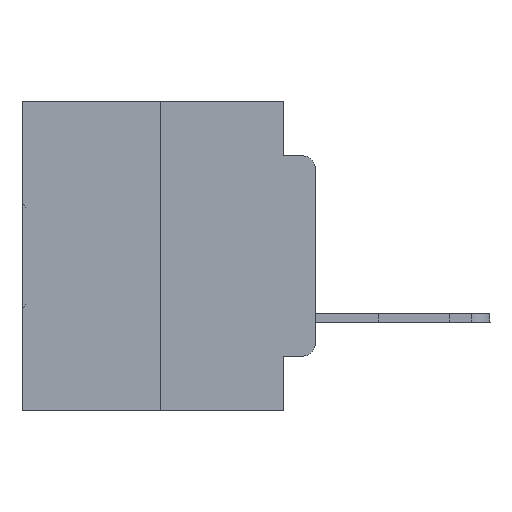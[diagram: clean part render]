
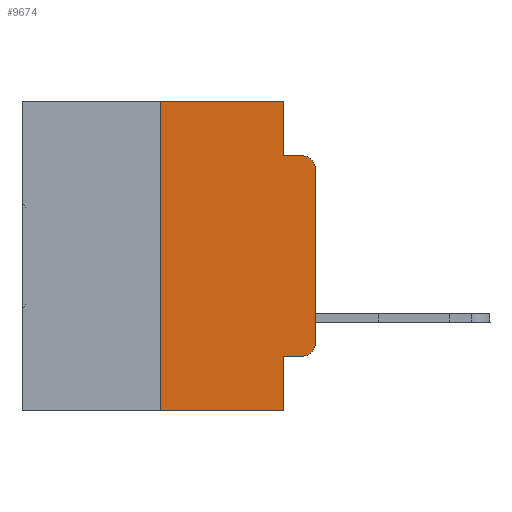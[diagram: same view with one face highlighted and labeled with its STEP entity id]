
A CAD part, left-side view. The second image highlights one B-rep face of the part: STEP entity #9674.
In plain terms, the highlighted planar face has unit normal (-1, 0, 0).
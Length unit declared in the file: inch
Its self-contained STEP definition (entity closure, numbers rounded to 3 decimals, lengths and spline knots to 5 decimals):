
#118 = ORIENTED_EDGE ( 'NONE', *, *, #8138, .T. ) ;
#133 = LINE ( 'NONE', #28961, #28469 ) ;
#849 = DIRECTION ( 'NONE',  ( -1., 0., 0. ) ) ;
#954 = DIRECTION ( 'NONE',  ( 0., 0., -1. ) ) ;
#1619 = CARTESIAN_POINT ( 'NONE',  ( 0., 0.473, 0. ) ) ;
#2212 = FACE_OUTER_BOUND ( 'NONE', #28470, .T. ) ;
#2397 = ORIENTED_EDGE ( 'NONE', *, *, #27612, .T. ) ;
#2568 = CIRCLE ( 'NONE', #22757, 0.02 ) ;
#2990 = VECTOR ( 'NONE', #17232, 39.37008 ) ;
#3203 = EDGE_CURVE ( 'NONE', #25493, #4615, #4268, .T. ) ;
#4016 = CARTESIAN_POINT ( 'NONE',  ( 0., 0.02, -0.4115 ) ) ;
#4268 = LINE ( 'NONE', #20964, #20093 ) ;
#4605 = VERTEX_POINT ( 'NONE', #16360 ) ;
#4615 = VERTEX_POINT ( 'NONE', #11891 ) ;
#5071 = VECTOR ( 'NONE', #20044, 39.37008 ) ;
#5284 = CARTESIAN_POINT ( 'NONE',  ( 0., 0.051, 0. ) ) ;
#5314 = EDGE_CURVE ( 'NONE', #11670, #20157, #16582, .T. ) ;
#5320 = ORIENTED_EDGE ( 'NONE', *, *, #5314, .T. ) ;
#6007 = CARTESIAN_POINT ( 'NONE',  ( 0., 0., -0.1085 ) ) ;
#6512 = DIRECTION ( 'NONE',  ( 0., 0., 1. ) ) ;
#6536 = VERTEX_POINT ( 'NONE', #9984 ) ;
#6671 = VERTEX_POINT ( 'NONE', #12027 ) ;
#7410 = CIRCLE ( 'NONE', #23079, 0.02 ) ;
#7825 = CARTESIAN_POINT ( 'NONE',  ( 0., 0.02, -0.1085 ) ) ;
#7965 = DIRECTION ( 'NONE',  ( 0., 0., -1. ) ) ;
#8040 = DIRECTION ( 'NONE',  ( 0., -1., 0. ) ) ;
#8138 = EDGE_CURVE ( 'NONE', #6536, #22049, #23464, .T. ) ;
#8354 = EDGE_CURVE ( 'NONE', #6671, #29490, #18527, .T. ) ;
#8698 = CARTESIAN_POINT ( 'NONE',  ( 0., 0.051, -0.5 ) ) ;
#8813 = DIRECTION ( 'NONE',  ( 0., -1., 0. ) ) ;
#9592 = EDGE_CURVE ( 'NONE', #20157, #6536, #2568, .T. ) ;
#9674 = ADVANCED_FACE ( 'NONE', ( #2212 ), #11490, .F. ) ;
#9708 = CARTESIAN_POINT ( 'NONE',  ( 0., 0., 0. ) ) ;
#9984 = CARTESIAN_POINT ( 'NONE',  ( 0., 0., -0.3915 ) ) ;
#10073 = DIRECTION ( 'NONE',  ( 0., -1., 0. ) ) ;
#10475 = VECTOR ( 'NONE', #8040, 39.37008 ) ;
#10512 = CARTESIAN_POINT ( 'NONE',  ( 0., 0.02, -0.3915 ) ) ;
#10734 = VERTEX_POINT ( 'NONE', #8698 ) ;
#10777 = CARTESIAN_POINT ( 'NONE',  ( 0., 0.051, -0.0885 ) ) ;
#10799 = DIRECTION ( 'NONE',  ( 1., 0., 0. ) ) ;
#10843 = AXIS2_PLACEMENT_3D ( 'NONE', #21805, #10799, #23010 ) ;
#11021 = ORIENTED_EDGE ( 'NONE', *, *, #9592, .T. ) ;
#11490 = PLANE ( 'NONE',  #10843 ) ;
#11670 = VERTEX_POINT ( 'NONE', #25630 ) ;
#11891 = CARTESIAN_POINT ( 'NONE',  ( 0., 0.25, 0. ) ) ;
#12027 = CARTESIAN_POINT ( 'NONE',  ( 0., 0.051, 0. ) ) ;
#13637 = LINE ( 'NONE', #15046, #2990 ) ;
#13674 = ORIENTED_EDGE ( 'NONE', *, *, #25780, .F. ) ;
#14343 = CARTESIAN_POINT ( 'NONE',  ( 0., 0.25, -0.5 ) ) ;
#14591 = ORIENTED_EDGE ( 'NONE', *, *, #18285, .F. ) ;
#15046 = CARTESIAN_POINT ( 'NONE',  ( 0., 0.473, -0.5 ) ) ;
#15161 = CARTESIAN_POINT ( 'NONE',  ( 0., 0.051, -0.4115 ) ) ;
#15295 = DIRECTION ( 'NONE',  ( -1., 0., 0. ) ) ;
#16360 = CARTESIAN_POINT ( 'NONE',  ( 0., 0.02, -0.0885 ) ) ;
#16582 = LINE ( 'NONE', #15161, #10475 ) ;
#16876 = VECTOR ( 'NONE', #8813, 39.37008 ) ;
#17232 = DIRECTION ( 'NONE',  ( 0., -1., 0. ) ) ;
#17324 = EDGE_CURVE ( 'NONE', #22049, #4605, #7410, .T. ) ;
#17903 = LINE ( 'NONE', #5284, #5071 ) ;
#18148 = VECTOR ( 'NONE', #7965, 39.37008 ) ;
#18285 = EDGE_CURVE ( 'NONE', #11670, #10734, #17903, .T. ) ;
#18527 = LINE ( 'NONE', #20007, #18148 ) ;
#19208 = DIRECTION ( 'NONE',  ( 0., 0., 1. ) ) ;
#20007 = CARTESIAN_POINT ( 'NONE',  ( 0., 0.051, 0. ) ) ;
#20044 = DIRECTION ( 'NONE',  ( 0., 0., -1. ) ) ;
#20093 = VECTOR ( 'NONE', #6512, 39.37008 ) ;
#20157 = VERTEX_POINT ( 'NONE', #4016 ) ;
#20816 = ORIENTED_EDGE ( 'NONE', *, *, #17324, .T. ) ;
#20964 = CARTESIAN_POINT ( 'NONE',  ( 0., 0.25, 0. ) ) ;
#21214 = VECTOR ( 'NONE', #19208, 39.37008 ) ;
#21520 = ORIENTED_EDGE ( 'NONE', *, *, #24732, .F. ) ;
#21805 = CARTESIAN_POINT ( 'NONE',  ( 0., 0.473, 0. ) ) ;
#22049 = VERTEX_POINT ( 'NONE', #6007 ) ;
#22757 = AXIS2_PLACEMENT_3D ( 'NONE', #10512, #15295, #25071 ) ;
#23010 = DIRECTION ( 'NONE',  ( 0., 0., -1. ) ) ;
#23079 = AXIS2_PLACEMENT_3D ( 'NONE', #7825, #849, #954 ) ;
#23464 = LINE ( 'NONE', #9708, #21214 ) ;
#24368 = LINE ( 'NONE', #1619, #16876 ) ;
#24732 = EDGE_CURVE ( 'NONE', #4615, #6671, #24368, .T. ) ;
#25071 = DIRECTION ( 'NONE',  ( 0., 0., -1. ) ) ;
#25493 = VERTEX_POINT ( 'NONE', #14343 ) ;
#25630 = CARTESIAN_POINT ( 'NONE',  ( 0., 0.051, -0.4115 ) ) ;
#25780 = EDGE_CURVE ( 'NONE', #29490, #4605, #133, .T. ) ;
#27612 = EDGE_CURVE ( 'NONE', #25493, #10734, #13637, .T. ) ;
#28469 = VECTOR ( 'NONE', #10073, 39.37008 ) ;
#28470 = EDGE_LOOP ( 'NONE', ( #118, #20816, #13674, #28839, #21520, #28680, #2397, #14591, #5320, #11021 ) ) ;
#28680 = ORIENTED_EDGE ( 'NONE', *, *, #3203, .F. ) ;
#28839 = ORIENTED_EDGE ( 'NONE', *, *, #8354, .F. ) ;
#28961 = CARTESIAN_POINT ( 'NONE',  ( 0., 0.051, -0.0885 ) ) ;
#29490 = VERTEX_POINT ( 'NONE', #10777 ) ;
